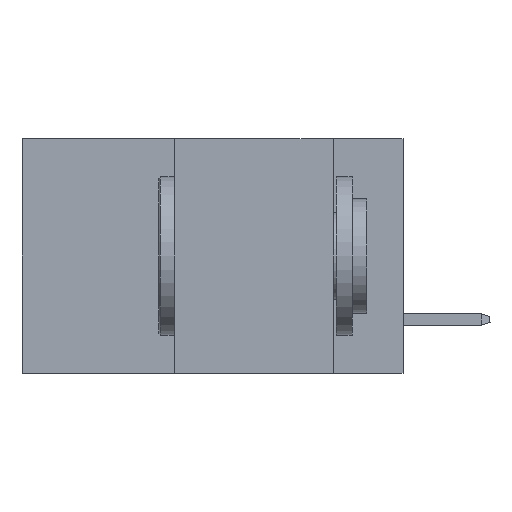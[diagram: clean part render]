
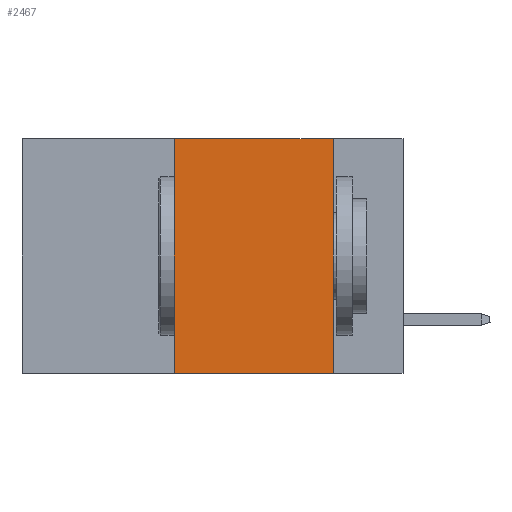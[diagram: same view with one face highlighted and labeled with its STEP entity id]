
A CAD part, left-side view. The second image highlights one B-rep face of the part: STEP entity #2467.
In plain terms, the highlighted planar face has unit normal (-1, 0, 0).
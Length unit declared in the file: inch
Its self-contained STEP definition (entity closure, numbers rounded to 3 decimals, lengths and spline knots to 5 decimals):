
#13 = FACE_OUTER_BOUND ( 'NONE', #4856, .T. ) ;
#237 = DIRECTION ( 'NONE',  ( 0., -1., 0. ) ) ;
#453 = CARTESIAN_POINT ( 'NONE',  ( 0., 0.6, -0.37 ) ) ;
#855 = CARTESIAN_POINT ( 'NONE',  ( 0., 0.36, 0. ) ) ;
#1272 = PLANE ( 'NONE',  #5764 ) ;
#1472 = LINE ( 'NONE', #6768, #15696 ) ;
#1910 = ORIENTED_EDGE ( 'NONE', *, *, #3753, .T. ) ;
#2409 = LINE ( 'NONE', #453, #8713 ) ;
#2467 = ADVANCED_FACE ( 'NONE', ( #13 ), #1272, .F. ) ;
#3204 = ORIENTED_EDGE ( 'NONE', *, *, #18288, .F. ) ;
#3753 = EDGE_CURVE ( 'NONE', #18703, #4522, #2409, .T. ) ;
#3954 = CARTESIAN_POINT ( 'NONE',  ( 0., 0.6, 0. ) ) ;
#4341 = VECTOR ( 'NONE', #8951, 39.37008 ) ;
#4522 = VERTEX_POINT ( 'NONE', #12269 ) ;
#4856 = EDGE_LOOP ( 'NONE', ( #7422, #16199, #3204, #1910 ) ) ;
#5764 = AXIS2_PLACEMENT_3D ( 'NONE', #15238, #7008, #19100 ) ;
#5786 = LINE ( 'NONE', #3954, #4341 ) ;
#6450 = LINE ( 'NONE', #6776, #12683 ) ;
#6768 = CARTESIAN_POINT ( 'NONE',  ( 0., 0.11, 0. ) ) ;
#6776 = CARTESIAN_POINT ( 'NONE',  ( 0., 0.36, 0. ) ) ;
#7008 = DIRECTION ( 'NONE',  ( 1., 0., 0. ) ) ;
#7422 = ORIENTED_EDGE ( 'NONE', *, *, #20458, .F. ) ;
#8713 = VECTOR ( 'NONE', #237, 39.37008 ) ;
#8951 = DIRECTION ( 'NONE',  ( 0., -1., 0. ) ) ;
#11579 = CARTESIAN_POINT ( 'NONE',  ( 0., 0.36, -0.37 ) ) ;
#12269 = CARTESIAN_POINT ( 'NONE',  ( 0., 0.11, -0.37 ) ) ;
#12683 = VECTOR ( 'NONE', #20384, 39.37008 ) ;
#13003 = VERTEX_POINT ( 'NONE', #855 ) ;
#13698 = VERTEX_POINT ( 'NONE', #17394 ) ;
#15238 = CARTESIAN_POINT ( 'NONE',  ( 0., 0.6, 0. ) ) ;
#15696 = VECTOR ( 'NONE', #20700, 39.37008 ) ;
#16199 = ORIENTED_EDGE ( 'NONE', *, *, #19695, .F. ) ;
#17394 = CARTESIAN_POINT ( 'NONE',  ( 0., 0.11, 0. ) ) ;
#18288 = EDGE_CURVE ( 'NONE', #18703, #13003, #6450, .T. ) ;
#18703 = VERTEX_POINT ( 'NONE', #11579 ) ;
#19100 = DIRECTION ( 'NONE',  ( 0., 0., -1. ) ) ;
#19695 = EDGE_CURVE ( 'NONE', #13003, #13698, #5786, .T. ) ;
#20384 = DIRECTION ( 'NONE',  ( 0., 0., 1. ) ) ;
#20458 = EDGE_CURVE ( 'NONE', #13698, #4522, #1472, .T. ) ;
#20700 = DIRECTION ( 'NONE',  ( 0., 0., -1. ) ) ;
